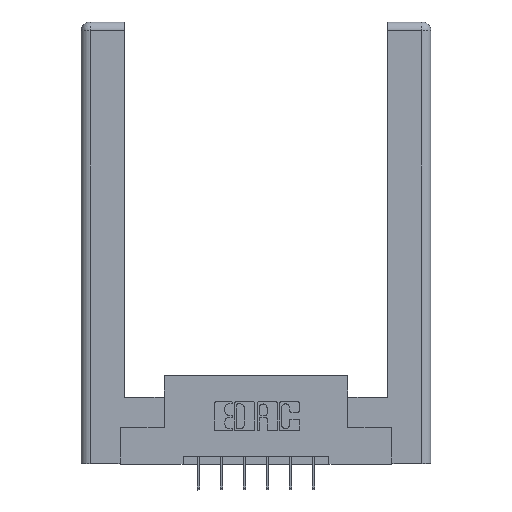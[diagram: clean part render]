
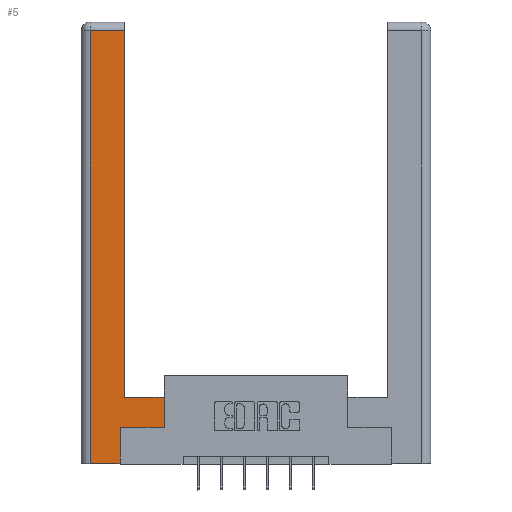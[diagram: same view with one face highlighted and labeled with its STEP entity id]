
A CAD part, top view. The second image highlights one B-rep face of the part: STEP entity #5.
In plain terms, the highlighted planar face has unit normal (0, 0, 1).
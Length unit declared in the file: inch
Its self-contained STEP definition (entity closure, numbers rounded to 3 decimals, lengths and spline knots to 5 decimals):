
#5 = ADVANCED_FACE ( 'NONE', ( #3295 ), #7047, .F. ) ;
#124 = CARTESIAN_POINT ( 'NONE',  ( 0.265, 0., 0. ) ) ;
#210 = CARTESIAN_POINT ( 'NONE',  ( 0.565, 0.45, 0. ) ) ;
#409 = LINE ( 'NONE', #5765, #6238 ) ;
#857 = CARTESIAN_POINT ( 'NONE',  ( 0.265, 0.245, 0. ) ) ;
#1350 = LINE ( 'NONE', #11820, #1640 ) ;
#1523 = CARTESIAN_POINT ( 'NONE',  ( 0., 0., 0. ) ) ;
#1640 = VECTOR ( 'NONE', #8121, 39.37008 ) ;
#1796 = VERTEX_POINT ( 'NONE', #2737 ) ;
#1911 = CARTESIAN_POINT ( 'NONE',  ( 0.295, 0.45, 0. ) ) ;
#1971 = LINE ( 'NONE', #210, #11576 ) ;
#2080 = DIRECTION ( 'NONE',  ( 0., 1., 0. ) ) ;
#2253 = EDGE_CURVE ( 'NONE', #9794, #5716, #8508, .T. ) ;
#2423 = EDGE_CURVE ( 'NONE', #7037, #9485, #4247, .T. ) ;
#2737 = CARTESIAN_POINT ( 'NONE',  ( 0.565, 0.45, 0. ) ) ;
#2823 = VECTOR ( 'NONE', #3492, 39.37008 ) ;
#3129 = CARTESIAN_POINT ( 'NONE',  ( 0.295, 2.94, 0. ) ) ;
#3295 = FACE_OUTER_BOUND ( 'NONE', #6224, .T. ) ;
#3296 = ORIENTED_EDGE ( 'NONE', *, *, #8157, .T. ) ;
#3332 = CARTESIAN_POINT ( 'NONE',  ( 0.565, 0.245, 0. ) ) ;
#3366 = VECTOR ( 'NONE', #10418, 39.37008 ) ;
#3367 = CARTESIAN_POINT ( 'NONE',  ( 0.565, 0.245, 0. ) ) ;
#3492 = DIRECTION ( 'NONE',  ( 1., 0., 0. ) ) ;
#3635 = CARTESIAN_POINT ( 'NONE',  ( 0.295, 0.45, 0. ) ) ;
#4247 = LINE ( 'NONE', #7335, #11986 ) ;
#4281 = ORIENTED_EDGE ( 'NONE', *, *, #10381, .T. ) ;
#4303 = DIRECTION ( 'NONE',  ( 0., 0., -1. ) ) ;
#4335 = EDGE_CURVE ( 'NONE', #9337, #6825, #8023, .T. ) ;
#5175 = CARTESIAN_POINT ( 'NONE',  ( 0.0615, 0., 0. ) ) ;
#5511 = VECTOR ( 'NONE', #7899, 39.37008 ) ;
#5657 = EDGE_CURVE ( 'NONE', #11781, #9794, #1350, .T. ) ;
#5716 = VERTEX_POINT ( 'NONE', #3332 ) ;
#5765 = CARTESIAN_POINT ( 'NONE',  ( 0.265, 0., 0. ) ) ;
#6186 = DIRECTION ( 'NONE',  ( -1., 0., 0. ) ) ;
#6224 = EDGE_LOOP ( 'NONE', ( #10563, #7593, #9144, #4281, #8629, #10915, #6908, #3296 ) ) ;
#6238 = VECTOR ( 'NONE', #7669, 39.37008 ) ;
#6452 = CARTESIAN_POINT ( 'NONE',  ( 0.0615, 2.94, 0. ) ) ;
#6656 = EDGE_CURVE ( 'NONE', #5716, #1796, #1971, .T. ) ;
#6825 = VERTEX_POINT ( 'NONE', #5175 ) ;
#6908 = ORIENTED_EDGE ( 'NONE', *, *, #6656, .T. ) ;
#7037 = VERTEX_POINT ( 'NONE', #3635 ) ;
#7047 = PLANE ( 'NONE',  #9994 ) ;
#7335 = CARTESIAN_POINT ( 'NONE',  ( 0.295, 3., 0. ) ) ;
#7593 = ORIENTED_EDGE ( 'NONE', *, *, #11592, .T. ) ;
#7669 = DIRECTION ( 'NONE',  ( 1., 0., 0. ) ) ;
#7705 = CARTESIAN_POINT ( 'NONE',  ( 0.0615, 2.94, 0. ) ) ;
#7899 = DIRECTION ( 'NONE',  ( 0., -1., 0. ) ) ;
#8023 = LINE ( 'NONE', #9860, #5511 ) ;
#8121 = DIRECTION ( 'NONE',  ( 0., 1., 0. ) ) ;
#8157 = EDGE_CURVE ( 'NONE', #1796, #7037, #11107, .T. ) ;
#8337 = DIRECTION ( 'NONE',  ( -1., 0., 0. ) ) ;
#8508 = LINE ( 'NONE', #3367, #2823 ) ;
#8629 = ORIENTED_EDGE ( 'NONE', *, *, #5657, .T. ) ;
#8843 = VECTOR ( 'NONE', #8337, 39.37008 ) ;
#9144 = ORIENTED_EDGE ( 'NONE', *, *, #4335, .T. ) ;
#9337 = VERTEX_POINT ( 'NONE', #7705 ) ;
#9485 = VERTEX_POINT ( 'NONE', #3129 ) ;
#9794 = VERTEX_POINT ( 'NONE', #857 ) ;
#9860 = CARTESIAN_POINT ( 'NONE',  ( 0.0615, 0., 0. ) ) ;
#9994 = AXIS2_PLACEMENT_3D ( 'NONE', #1523, #4303, #6186 ) ;
#10146 = DIRECTION ( 'NONE',  ( 0., 1., 0. ) ) ;
#10381 = EDGE_CURVE ( 'NONE', #6825, #11781, #409, .T. ) ;
#10418 = DIRECTION ( 'NONE',  ( -1., 0., 0. ) ) ;
#10563 = ORIENTED_EDGE ( 'NONE', *, *, #2423, .T. ) ;
#10915 = ORIENTED_EDGE ( 'NONE', *, *, #2253, .T. ) ;
#11107 = LINE ( 'NONE', #1911, #3366 ) ;
#11576 = VECTOR ( 'NONE', #2080, 39.37008 ) ;
#11592 = EDGE_CURVE ( 'NONE', #9485, #9337, #11610, .T. ) ;
#11610 = LINE ( 'NONE', #6452, #8843 ) ;
#11781 = VERTEX_POINT ( 'NONE', #124 ) ;
#11820 = CARTESIAN_POINT ( 'NONE',  ( 0.265, 0.245, 0. ) ) ;
#11986 = VECTOR ( 'NONE', #10146, 39.37008 ) ;
